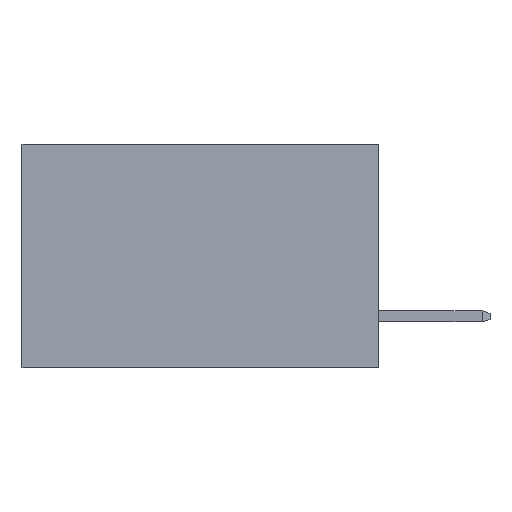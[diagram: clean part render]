
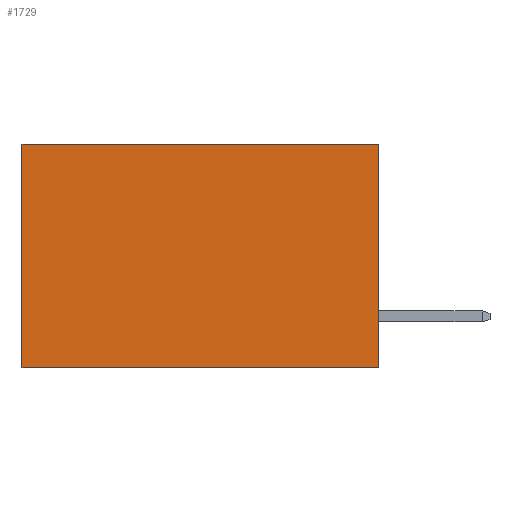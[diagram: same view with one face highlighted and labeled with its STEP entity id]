
A CAD part, left-side view. The second image highlights one B-rep face of the part: STEP entity #1729.
In plain terms, the highlighted planar face has unit normal (-1, 0, 0).
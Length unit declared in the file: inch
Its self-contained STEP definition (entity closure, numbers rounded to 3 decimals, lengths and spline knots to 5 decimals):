
#396 = VECTOR ( 'NONE', #6405, 39.37008 ) ;
#1729 = ADVANCED_FACE ( 'NONE', ( #9759 ), #2888, .F. ) ;
#2589 = VERTEX_POINT ( 'NONE', #7294 ) ;
#2888 = PLANE ( 'NONE',  #25327 ) ;
#2948 = CARTESIAN_POINT ( 'NONE',  ( 0.277, 0., -0.37 ) ) ;
#3250 = VECTOR ( 'NONE', #9570, 39.37008 ) ;
#3733 = DIRECTION ( 'NONE',  ( 0., 0., -1. ) ) ;
#3738 = EDGE_LOOP ( 'NONE', ( #21829, #15641, #19636, #4693 ) ) ;
#3776 = VECTOR ( 'NONE', #16877, 39.37008 ) ;
#4445 = VECTOR ( 'NONE', #19522, 39.37008 ) ;
#4548 = LINE ( 'NONE', #6513, #396 ) ;
#4558 = CARTESIAN_POINT ( 'NONE',  ( 0.277, 0., -0.37 ) ) ;
#4693 = ORIENTED_EDGE ( 'NONE', *, *, #5563, .T. ) ;
#5463 = CARTESIAN_POINT ( 'NONE',  ( 0.277, 0.59, 0. ) ) ;
#5563 = EDGE_CURVE ( 'NONE', #6192, #9905, #4548, .T. ) ;
#6192 = VERTEX_POINT ( 'NONE', #13576 ) ;
#6405 = DIRECTION ( 'NONE',  ( 0., 1., 0. ) ) ;
#6513 = CARTESIAN_POINT ( 'NONE',  ( 0.277, 0., 0. ) ) ;
#7294 = CARTESIAN_POINT ( 'NONE',  ( 0.277, 0.59, -0.37 ) ) ;
#9570 = DIRECTION ( 'NONE',  ( 0., 0., -1. ) ) ;
#9759 = FACE_OUTER_BOUND ( 'NONE', #3738, .T. ) ;
#9905 = VERTEX_POINT ( 'NONE', #5463 ) ;
#10614 = EDGE_CURVE ( 'NONE', #6192, #15566, #20356, .T. ) ;
#13576 = CARTESIAN_POINT ( 'NONE',  ( 0.277, 0., 0. ) ) ;
#14339 = LINE ( 'NONE', #14880, #3776 ) ;
#14880 = CARTESIAN_POINT ( 'NONE',  ( 0.277, 0., -0.37 ) ) ;
#15566 = VERTEX_POINT ( 'NONE', #4558 ) ;
#15641 = ORIENTED_EDGE ( 'NONE', *, *, #18237, .F. ) ;
#16535 = EDGE_CURVE ( 'NONE', #9905, #2589, #24386, .T. ) ;
#16877 = DIRECTION ( 'NONE',  ( 0., 1., 0. ) ) ;
#18237 = EDGE_CURVE ( 'NONE', #15566, #2589, #14339, .T. ) ;
#19493 = CARTESIAN_POINT ( 'NONE',  ( 0.277, 0.59, -0.37 ) ) ;
#19522 = DIRECTION ( 'NONE',  ( 0., 0., -1. ) ) ;
#19636 = ORIENTED_EDGE ( 'NONE', *, *, #10614, .F. ) ;
#19991 = DIRECTION ( 'NONE',  ( 1., 0., 0. ) ) ;
#20356 = LINE ( 'NONE', #21481, #4445 ) ;
#21481 = CARTESIAN_POINT ( 'NONE',  ( 0.277, 0., -0.37 ) ) ;
#21829 = ORIENTED_EDGE ( 'NONE', *, *, #16535, .T. ) ;
#24386 = LINE ( 'NONE', #19493, #3250 ) ;
#25327 = AXIS2_PLACEMENT_3D ( 'NONE', #2948, #19991, #3733 ) ;
